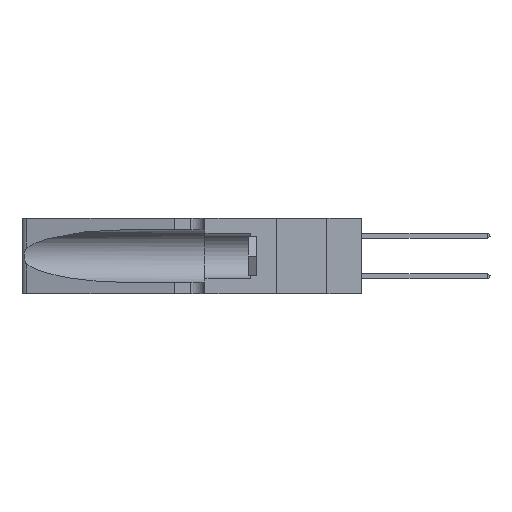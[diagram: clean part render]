
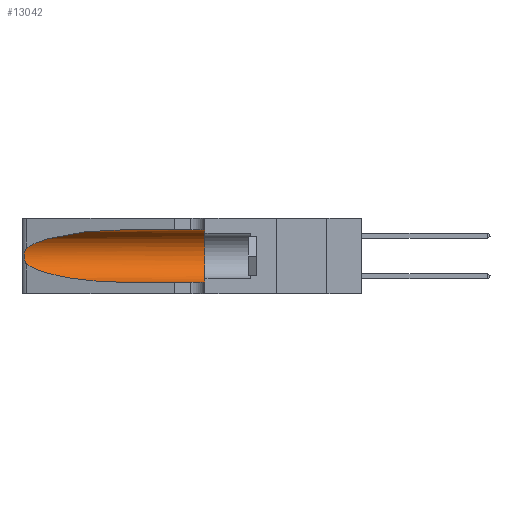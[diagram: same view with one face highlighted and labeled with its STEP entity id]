
A CAD part, left-side view. The second image highlights one B-rep face of the part: STEP entity #13042.
In plain terms, the highlighted cylindrical face has radius 3.308 mm (diameter 6.617 mm), a partial arc.
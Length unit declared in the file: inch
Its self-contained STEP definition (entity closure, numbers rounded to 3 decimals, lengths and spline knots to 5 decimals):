
#88 = VECTOR ( 'NONE', #9729, 39.37008 ) ;
#338 = CARTESIAN_POINT ( 'NONE',  ( 0.25487, 1.22718, 0.22369 ) ) ;
#345 = CARTESIAN_POINT ( 'NONE',  ( 0.2373, 1.15595, 0.28018 ) ) ;
#420 = VERTEX_POINT ( 'NONE', #3716 ) ;
#422 = CARTESIAN_POINT ( 'NONE',  ( 0.25487, 1.22718, 0.14631 ) ) ;
#951 = ORIENTED_EDGE ( 'NONE', *, *, #8011, .F. ) ;
#1341 = CARTESIAN_POINT ( 'NONE',  ( 0.1305, 1.61858, 0.31525 ) ) ;
#1878 = AXIS2_PLACEMENT_3D ( 'NONE', #7774, #13167, #16769 ) ;
#2247 = CARTESIAN_POINT ( 'NONE',  ( 0.25639, 1.23184, 0.21858 ) ) ;
#2256 = CARTESIAN_POINT ( 'NONE',  ( 0.18966, 0.96281, 0.31525 ) ) ;
#2684 = ORIENTED_EDGE ( 'NONE', *, *, #16580, .T. ) ;
#2922 = EDGE_CURVE ( 'NONE', #9882, #13566, #23528, .T. ) ;
#3716 = CARTESIAN_POINT ( 'NONE',  ( 0.1305, 0.35, 0.31525 ) ) ;
#3781 = EDGE_CURVE ( 'NONE', #18049, #9884, #15106, .T. ) ;
#4077 = CARTESIAN_POINT ( 'NONE',  ( 0.25854, 1.2359, 0.20912 ) ) ;
#4703 = DIRECTION ( 'NONE',  ( 0., 1., 0. ) ) ;
#5313 = CARTESIAN_POINT ( 'NONE',  ( 0.1305, 0.72297, 0.05475 ) ) ;
#5905 = CARTESIAN_POINT ( 'NONE',  ( 0.26075, 1.23896, 0.19203 ) ) ;
#6288 = CYLINDRICAL_SURFACE ( 'NONE', #1878, 0.13025 ) ;
#7056 = AXIS2_PLACEMENT_3D ( 'NONE', #15553, #4703, #17381 ) ;
#7752 = CARTESIAN_POINT ( 'NONE',  ( 0.26017, 1.23833, 0.17102 ) ) ;
#7774 = CARTESIAN_POINT ( 'NONE',  ( 0.1305, 1.61858, 0.185 ) ) ;
#7929 = CARTESIAN_POINT ( 'NONE',  ( 0.1305, 1.61858, 0.05475 ) ) ;
#8011 = EDGE_CURVE ( 'NONE', #18049, #420, #23155, .T. ) ;
#8354 = CIRCLE ( 'NONE', #7056, 0.13025 ) ;
#8547 = DIRECTION ( 'NONE',  ( 0., -1., 0. ) ) ;
#8897 = CARTESIAN_POINT ( 'NONE',  ( 0.25487, 1.22718, 0.14631 ) ) ;
#9155 = B_SPLINE_CURVE_WITH_KNOTS ( 'NONE', 3,
 ( #338, #22144, #2247, #14939, #4077, #16750, #5905, #18568, #7752, #20380, #9562, #22217, #11394, #422 ),
 .UNSPECIFIED., .F., .F.,
 ( 4, 2, 2, 2, 2, 2, 4 ),
 ( 0., 0.00027, 0.00053, 0.00107, 0.0016, 0.00187, 0.00214 ),
 .UNSPECIFIED. ) ;
#9562 = CARTESIAN_POINT ( 'NONE',  ( 0.25789, 1.23486, 0.15765 ) ) ;
#9729 = DIRECTION ( 'NONE',  ( 0., -1., 0. ) ) ;
#9882 = VERTEX_POINT ( 'NONE', #18876 ) ;
#9884 = VERTEX_POINT ( 'NONE', #20695 ) ;
#11322 = VERTEX_POINT ( 'NONE', #14106 ) ;
#11394 = CARTESIAN_POINT ( 'NONE',  ( 0.25555, 1.22993, 0.14849 ) ) ;
#11874 = EDGE_CURVE ( 'NONE', #420, #11322, #8354, .T. ) ;
#12380 = ORIENTED_EDGE ( 'NONE', *, *, #2922, .T. ) ;
#13042 = ADVANCED_FACE ( 'NONE', ( #20718 ), #6288, .F. ) ;
#13157 = CARTESIAN_POINT ( 'NONE',  ( 0.1305, 0.72297, 0.31525 ) ) ;
#13167 = DIRECTION ( 'NONE',  ( 0., -1., 0. ) ) ;
#13566 = VERTEX_POINT ( 'NONE', #18162 ) ;
#13880 = EDGE_LOOP ( 'NONE', ( #16854, #2684, #12380, #20285, #17264, #951 ) ) ;
#14106 = CARTESIAN_POINT ( 'NONE',  ( 0.1305, 0.35, 0.05475 ) ) ;
#14369 = CARTESIAN_POINT ( 'NONE',  ( 0.2373, 1.15595, 0.08982 ) ) ;
#14939 = CARTESIAN_POINT ( 'NONE',  ( 0.25787, 1.23484, 0.2124 ) ) ;
#15092 = EDGE_CURVE ( 'NONE', #13566, #11322, #18890, .T. ) ;
#15106 =( BOUNDED_CURVE ( )  B_SPLINE_CURVE ( 3, ( #13157, #2256, #345, #16761 ),
 .UNSPECIFIED., .F., .T. ) 
 B_SPLINE_CURVE_WITH_KNOTS ( ( 4, 4 ),
 ( 1.5708, 2.84003 ),
 .UNSPECIFIED. ) 
 CURVE ( )  GEOMETRIC_REPRESENTATION_ITEM ( )  RATIONAL_B_SPLINE_CURVE ( ( 1., 0.87, 0.87, 1. ) ) 
 REPRESENTATION_ITEM ( '' )  );
#15418 = CARTESIAN_POINT ( 'NONE',  ( 0.1305, 0.72297, 0.31525 ) ) ;
#15553 = CARTESIAN_POINT ( 'NONE',  ( 0.1305, 0.35, 0.185 ) ) ;
#16171 = CARTESIAN_POINT ( 'NONE',  ( 0.18966, 0.96281, 0.05475 ) ) ;
#16580 = EDGE_CURVE ( 'NONE', #9884, #9882, #9155, .T. ) ;
#16750 = CARTESIAN_POINT ( 'NONE',  ( 0.26018, 1.23835, 0.19895 ) ) ;
#16761 = CARTESIAN_POINT ( 'NONE',  ( 0.25487, 1.22718, 0.22369 ) ) ;
#16769 = DIRECTION ( 'NONE',  ( 0., 0., -1. ) ) ;
#16854 = ORIENTED_EDGE ( 'NONE', *, *, #3781, .T. ) ;
#17264 = ORIENTED_EDGE ( 'NONE', *, *, #11874, .F. ) ;
#17381 = DIRECTION ( 'NONE',  ( 0., 0., 1. ) ) ;
#17762 = VECTOR ( 'NONE', #8547, 39.37008 ) ;
#18049 = VERTEX_POINT ( 'NONE', #15418 ) ;
#18162 = CARTESIAN_POINT ( 'NONE',  ( 0.1305, 0.72297, 0.05475 ) ) ;
#18568 = CARTESIAN_POINT ( 'NONE',  ( 0.26075, 1.23896, 0.178 ) ) ;
#18876 = CARTESIAN_POINT ( 'NONE',  ( 0.25487, 1.22718, 0.14631 ) ) ;
#18890 = LINE ( 'NONE', #7929, #88 ) ;
#20285 = ORIENTED_EDGE ( 'NONE', *, *, #15092, .T. ) ;
#20380 = CARTESIAN_POINT ( 'NONE',  ( 0.25856, 1.23593, 0.16098 ) ) ;
#20695 = CARTESIAN_POINT ( 'NONE',  ( 0.25487, 1.22718, 0.22369 ) ) ;
#20718 = FACE_OUTER_BOUND ( 'NONE', #13880, .T. ) ;
#22144 = CARTESIAN_POINT ( 'NONE',  ( 0.25555, 1.22994, 0.2215 ) ) ;
#22217 = CARTESIAN_POINT ( 'NONE',  ( 0.25639, 1.23186, 0.15144 ) ) ;
#23155 = LINE ( 'NONE', #1341, #17762 ) ;
#23528 =( BOUNDED_CURVE ( )  B_SPLINE_CURVE ( 3, ( #8897, #14369, #16171, #5313 ),
 .UNSPECIFIED., .F., .F. ) 
 B_SPLINE_CURVE_WITH_KNOTS ( ( 4, 4 ),
 ( 3.44316, 4.71239 ),
 .UNSPECIFIED. ) 
 CURVE ( )  GEOMETRIC_REPRESENTATION_ITEM ( )  RATIONAL_B_SPLINE_CURVE ( ( 1., 0.87, 0.87, 1. ) ) 
 REPRESENTATION_ITEM ( '' )  );
